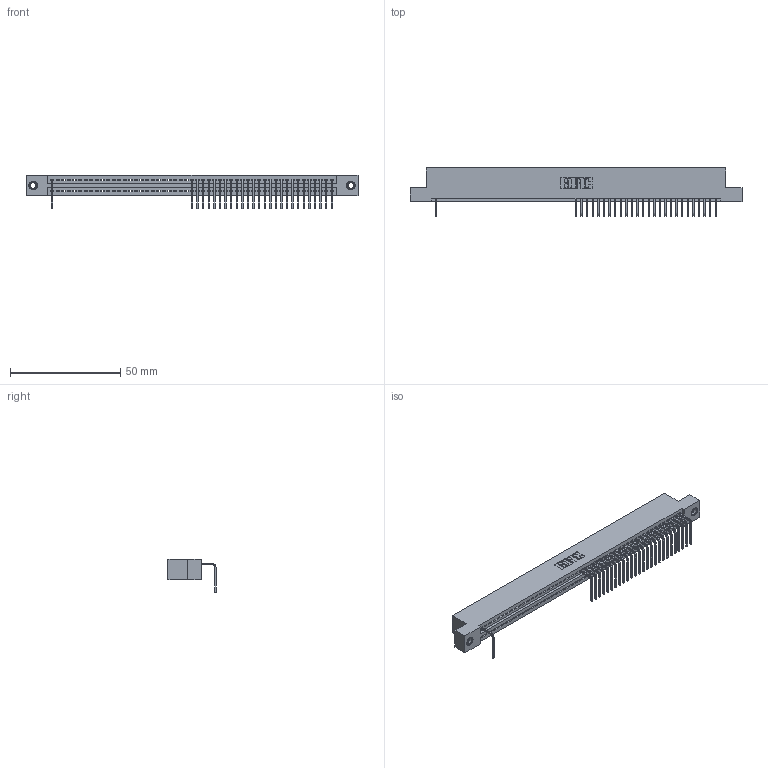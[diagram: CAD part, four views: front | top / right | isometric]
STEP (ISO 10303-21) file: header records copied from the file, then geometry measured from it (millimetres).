
FILE_DESCRIPTION (( 'STEP AP203' ), '1' );
FILE_NAME ('345-051-558-107.STEP', '2018-09-22T18:30:18', ( '' ), ( '' ), 'SwSTEP 2.0', 'SolidWorks 2016', '' );
FILE_SCHEMA (( 'CONFIG_CONTROL_DESIGN' ));
Length unit declared in the file: inch
Products named in the file (4): 345 Part_Flush Mounting Lugs - 0.156 Dia-TI; 345-292-001_558 Tail - 2; 345-250-001_345-250-005-103; 345-051-558-107
Assembly tree (30 placements, depth 2):
  345-051-558-107
    345 Part_Flush Mounting Lugs - 0.156 Dia-TI
    345-292-001_558 Tail - 2  x27
    345-250-001_345-250-005-103  x2
Bounding box: 150.75 x 21.83 x 15.37 mm (x, y, z)
Volume: 14193.6 mm3; surface area: 18086.1 mm2
Topology: 30 solids, 30 shells, 2190 faces, 6687 edges, 4414 vertices
Faces by surface type: plane 1582, cylinder 592, cone 12, torus 4
Entity records: 37674 total; most frequent: ORIENTED_EDGE 6618, CARTESIAN_POINT 6616, DIRECTION 5765, EDGE_CURVE 3309, VECTOR 2953, LINE 2953, VERTEX_POINT 2200, AXIS2_PLACEMENT_3D 1406
